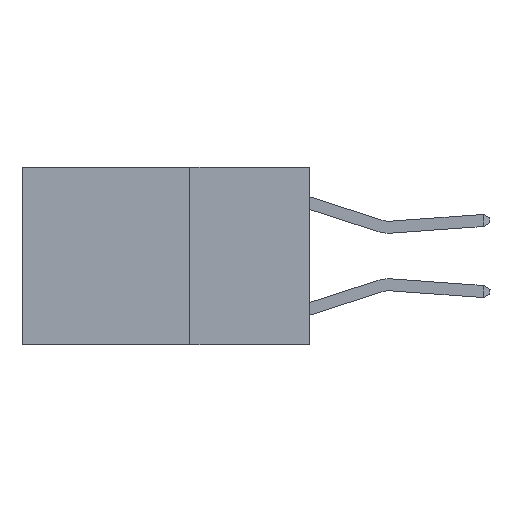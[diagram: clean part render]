
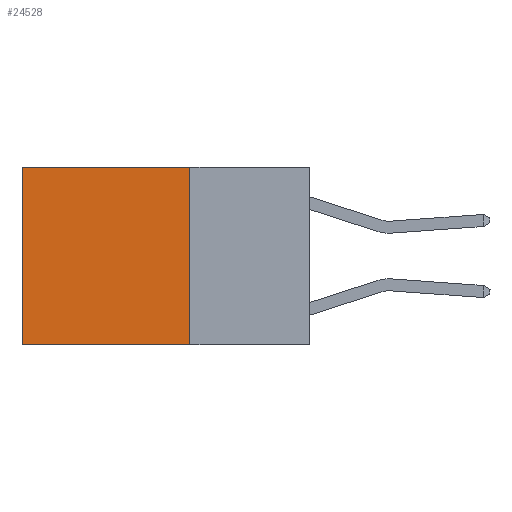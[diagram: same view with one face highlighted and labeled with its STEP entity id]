
A CAD part, left-side view. The second image highlights one B-rep face of the part: STEP entity #24528.
In plain terms, the highlighted planar face has unit normal (-1, 0, 0).
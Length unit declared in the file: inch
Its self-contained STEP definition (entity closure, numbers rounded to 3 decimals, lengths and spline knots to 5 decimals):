
#2017 = DIRECTION ( 'NONE',  ( 0., 1., 0. ) ) ;
#2351 = CARTESIAN_POINT ( 'NONE',  ( 0.2625, 0.25, 0. ) ) ;
#2614 = VECTOR ( 'NONE', #13691, 39.37008 ) ;
#3108 = VECTOR ( 'NONE', #2017, 39.37008 ) ;
#3291 = VECTOR ( 'NONE', #13112, 39.37008 ) ;
#3698 = VERTEX_POINT ( 'NONE', #2351 ) ;
#3981 = DIRECTION ( 'NONE',  ( 1., 0., 0. ) ) ;
#4034 = EDGE_CURVE ( 'NONE', #3698, #9946, #9856, .T. ) ;
#4860 = ORIENTED_EDGE ( 'NONE', *, *, #8296, .T. ) ;
#5429 = VERTEX_POINT ( 'NONE', #24529 ) ;
#5485 = DIRECTION ( 'NONE',  ( 0., 0., -1. ) ) ;
#5665 = LINE ( 'NONE', #7395, #19269 ) ;
#5955 = CARTESIAN_POINT ( 'NONE',  ( 0.2625, 0.25, -0.37 ) ) ;
#6366 = ORIENTED_EDGE ( 'NONE', *, *, #4034, .T. ) ;
#6594 = LINE ( 'NONE', #11750, #2614 ) ;
#7395 = CARTESIAN_POINT ( 'NONE',  ( 0.2625, 0.25, 0. ) ) ;
#8154 = EDGE_CURVE ( 'NONE', #3698, #11603, #5665, .T. ) ;
#8296 = EDGE_CURVE ( 'NONE', #9946, #5429, #6594, .T. ) ;
#8702 = FACE_OUTER_BOUND ( 'NONE', #11063, .T. ) ;
#8950 = ORIENTED_EDGE ( 'NONE', *, *, #10583, .F. ) ;
#8961 = LINE ( 'NONE', #5955, #3108 ) ;
#9856 = LINE ( 'NONE', #24432, #3291 ) ;
#9946 = VERTEX_POINT ( 'NONE', #11983 ) ;
#10583 = EDGE_CURVE ( 'NONE', #11603, #5429, #8961, .T. ) ;
#11063 = EDGE_LOOP ( 'NONE', ( #4860, #8950, #23380, #6366 ) ) ;
#11603 = VERTEX_POINT ( 'NONE', #22643 ) ;
#11750 = CARTESIAN_POINT ( 'NONE',  ( 0.2625, 0.6, 0. ) ) ;
#11759 = PLANE ( 'NONE',  #17387 ) ;
#11983 = CARTESIAN_POINT ( 'NONE',  ( 0.2625, 0.6, 0. ) ) ;
#13112 = DIRECTION ( 'NONE',  ( 0., 1., 0. ) ) ;
#13691 = DIRECTION ( 'NONE',  ( 0., 0., -1. ) ) ;
#15580 = CARTESIAN_POINT ( 'NONE',  ( 0.2625, 0.25, 0. ) ) ;
#17387 = AXIS2_PLACEMENT_3D ( 'NONE', #15580, #3981, #17547 ) ;
#17547 = DIRECTION ( 'NONE',  ( 0., 0., -1. ) ) ;
#19269 = VECTOR ( 'NONE', #5485, 39.37008 ) ;
#22643 = CARTESIAN_POINT ( 'NONE',  ( 0.2625, 0.25, -0.37 ) ) ;
#23380 = ORIENTED_EDGE ( 'NONE', *, *, #8154, .F. ) ;
#24432 = CARTESIAN_POINT ( 'NONE',  ( 0.2625, 0.25, 0. ) ) ;
#24528 = ADVANCED_FACE ( 'NONE', ( #8702 ), #11759, .F. ) ;
#24529 = CARTESIAN_POINT ( 'NONE',  ( 0.2625, 0.6, -0.37 ) ) ;
